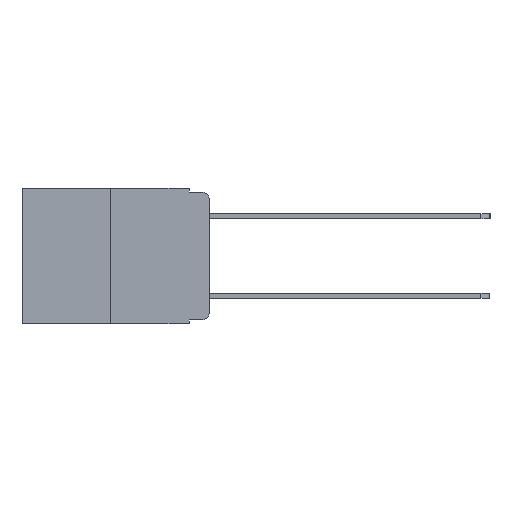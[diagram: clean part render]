
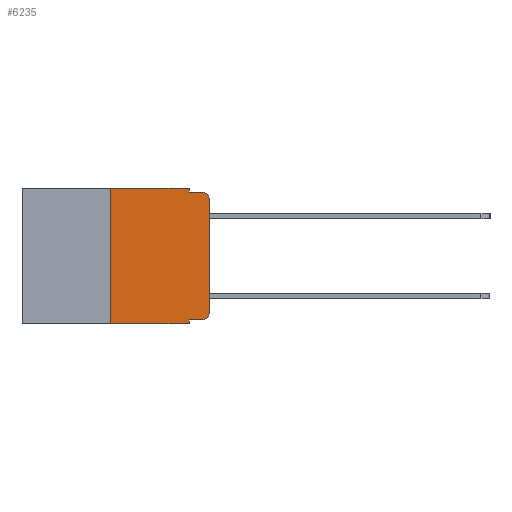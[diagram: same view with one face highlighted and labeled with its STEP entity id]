
A CAD part, left-side view. The second image highlights one B-rep face of the part: STEP entity #6235.
In plain terms, the highlighted planar face has unit normal (-1, 0, 0).
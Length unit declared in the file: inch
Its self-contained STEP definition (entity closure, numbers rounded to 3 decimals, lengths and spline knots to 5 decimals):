
#207 = LINE ( 'NONE', #10707, #4652 ) ;
#320 = VERTEX_POINT ( 'NONE', #2569 ) ;
#381 = CARTESIAN_POINT ( 'NONE',  ( 0., 0., -0.313 ) ) ;
#539 = ORIENTED_EDGE ( 'NONE', *, *, #3179, .T. ) ;
#1156 = EDGE_CURVE ( 'NONE', #10410, #8914, #207, .T. ) ;
#1241 = DIRECTION ( 'NONE',  ( 0., 0., 1. ) ) ;
#1415 = DIRECTION ( 'NONE',  ( 1., 0., 0. ) ) ;
#1929 = LINE ( 'NONE', #7719, #8649 ) ;
#2068 = DIRECTION ( 'NONE',  ( -1., 0., 0. ) ) ;
#2168 = CARTESIAN_POINT ( 'NONE',  ( 0., 0.25, -0.343 ) ) ;
#2192 = CARTESIAN_POINT ( 'NONE',  ( 0., 0.25, 0. ) ) ;
#2470 = DIRECTION ( 'NONE',  ( 0., -1., 0. ) ) ;
#2569 = CARTESIAN_POINT ( 'NONE',  ( 0., 0.25, 0. ) ) ;
#2578 = VERTEX_POINT ( 'NONE', #7697 ) ;
#2608 = CARTESIAN_POINT ( 'NONE',  ( 0., 0.051, -0.333 ) ) ;
#2634 = VECTOR ( 'NONE', #7077, 39.37008 ) ;
#2664 = ORIENTED_EDGE ( 'NONE', *, *, #4333, .T. ) ;
#2998 = VERTEX_POINT ( 'NONE', #6364 ) ;
#3070 = LINE ( 'NONE', #8947, #7781 ) ;
#3168 = CARTESIAN_POINT ( 'NONE',  ( 0., 0.473, 0. ) ) ;
#3179 = EDGE_CURVE ( 'NONE', #4422, #10410, #3642, .T. ) ;
#3642 = CIRCLE ( 'NONE', #3934, 0.02 ) ;
#3810 = VECTOR ( 'NONE', #8010, 39.37008 ) ;
#3842 = VECTOR ( 'NONE', #9845, 39.37008 ) ;
#3934 = AXIS2_PLACEMENT_3D ( 'NONE', #5834, #5812, #5856 ) ;
#4007 = VECTOR ( 'NONE', #2470, 39.37008 ) ;
#4014 = PLANE ( 'NONE',  #9168 ) ;
#4079 = VERTEX_POINT ( 'NONE', #2168 ) ;
#4333 = EDGE_CURVE ( 'NONE', #9180, #4422, #6713, .T. ) ;
#4422 = VERTEX_POINT ( 'NONE', #9756 ) ;
#4426 = VERTEX_POINT ( 'NONE', #9611 ) ;
#4652 = VECTOR ( 'NONE', #9319, 39.37008 ) ;
#4984 = DIRECTION ( 'NONE',  ( 0., -1., 0. ) ) ;
#5151 = FACE_OUTER_BOUND ( 'NONE', #6598, .T. ) ;
#5559 = EDGE_CURVE ( 'NONE', #9180, #2578, #9285, .T. ) ;
#5779 = CARTESIAN_POINT ( 'NONE',  ( 0., 0.051, -0.333 ) ) ;
#5812 = DIRECTION ( 'NONE',  ( -1., 0., 0. ) ) ;
#5834 = CARTESIAN_POINT ( 'NONE',  ( 0., 0.02, -0.313 ) ) ;
#5856 = DIRECTION ( 'NONE',  ( 0., 0., -1. ) ) ;
#6220 = LINE ( 'NONE', #11119, #3810 ) ;
#6235 = ADVANCED_FACE ( 'NONE', ( #5151 ), #4014, .F. ) ;
#6253 = LINE ( 'NONE', #10564, #3842 ) ;
#6299 = ORIENTED_EDGE ( 'NONE', *, *, #1156, .T. ) ;
#6364 = CARTESIAN_POINT ( 'NONE',  ( 0., 0.02, -0.01 ) ) ;
#6561 = CARTESIAN_POINT ( 'NONE',  ( 0., 0.051, -0.01 ) ) ;
#6563 = EDGE_CURVE ( 'NONE', #320, #4426, #3070, .T. ) ;
#6573 = ORIENTED_EDGE ( 'NONE', *, *, #11093, .T. ) ;
#6598 = EDGE_LOOP ( 'NONE', ( #6299, #6573, #7975, #8119, #6860, #8892, #10403, #11112, #2664, #539 ) ) ;
#6713 = LINE ( 'NONE', #5779, #4007 ) ;
#6771 = EDGE_CURVE ( 'NONE', #4079, #320, #10524, .T. ) ;
#6860 = ORIENTED_EDGE ( 'NONE', *, *, #6563, .F. ) ;
#7077 = DIRECTION ( 'NONE',  ( 0., 0., -1. ) ) ;
#7386 = CARTESIAN_POINT ( 'NONE',  ( 0., 0.02, -0.03 ) ) ;
#7618 = CARTESIAN_POINT ( 'NONE',  ( 0., 0., -0.03 ) ) ;
#7639 = DIRECTION ( 'NONE',  ( 0., 0., -1. ) ) ;
#7697 = CARTESIAN_POINT ( 'NONE',  ( 0., 0.051, -0.343 ) ) ;
#7719 = CARTESIAN_POINT ( 'NONE',  ( 0., 0.473, -0.343 ) ) ;
#7781 = VECTOR ( 'NONE', #8159, 39.37008 ) ;
#7889 = AXIS2_PLACEMENT_3D ( 'NONE', #7386, #2068, #8253 ) ;
#7907 = EDGE_CURVE ( 'NONE', #4079, #2578, #1929, .T. ) ;
#7975 = ORIENTED_EDGE ( 'NONE', *, *, #10061, .F. ) ;
#8010 = DIRECTION ( 'NONE',  ( 0., -1., 0. ) ) ;
#8119 = ORIENTED_EDGE ( 'NONE', *, *, #8481, .F. ) ;
#8159 = DIRECTION ( 'NONE',  ( 0., -1., 0. ) ) ;
#8253 = DIRECTION ( 'NONE',  ( 0., 0., -1. ) ) ;
#8481 = EDGE_CURVE ( 'NONE', #4426, #10551, #6253, .T. ) ;
#8649 = VECTOR ( 'NONE', #4984, 39.37008 ) ;
#8892 = ORIENTED_EDGE ( 'NONE', *, *, #6771, .F. ) ;
#8914 = VERTEX_POINT ( 'NONE', #7618 ) ;
#8947 = CARTESIAN_POINT ( 'NONE',  ( 0., 0.473, 0. ) ) ;
#9168 = AXIS2_PLACEMENT_3D ( 'NONE', #3168, #1415, #7639 ) ;
#9180 = VERTEX_POINT ( 'NONE', #2608 ) ;
#9181 = VECTOR ( 'NONE', #1241, 39.37008 ) ;
#9285 = LINE ( 'NONE', #11069, #2634 ) ;
#9319 = DIRECTION ( 'NONE',  ( 0., 0., 1. ) ) ;
#9611 = CARTESIAN_POINT ( 'NONE',  ( 0., 0.051, 0. ) ) ;
#9756 = CARTESIAN_POINT ( 'NONE',  ( 0., 0.02, -0.333 ) ) ;
#9845 = DIRECTION ( 'NONE',  ( 0., 0., -1. ) ) ;
#10061 = EDGE_CURVE ( 'NONE', #10551, #2998, #6220, .T. ) ;
#10332 = CIRCLE ( 'NONE', #7889, 0.02 ) ;
#10403 = ORIENTED_EDGE ( 'NONE', *, *, #7907, .T. ) ;
#10410 = VERTEX_POINT ( 'NONE', #381 ) ;
#10524 = LINE ( 'NONE', #2192, #9181 ) ;
#10551 = VERTEX_POINT ( 'NONE', #6561 ) ;
#10564 = CARTESIAN_POINT ( 'NONE',  ( 0., 0.051, 0. ) ) ;
#10707 = CARTESIAN_POINT ( 'NONE',  ( 0., 0., 0. ) ) ;
#11069 = CARTESIAN_POINT ( 'NONE',  ( 0., 0.051, 0. ) ) ;
#11093 = EDGE_CURVE ( 'NONE', #8914, #2998, #10332, .T. ) ;
#11112 = ORIENTED_EDGE ( 'NONE', *, *, #5559, .F. ) ;
#11119 = CARTESIAN_POINT ( 'NONE',  ( 0., 0.051, -0.01 ) ) ;
